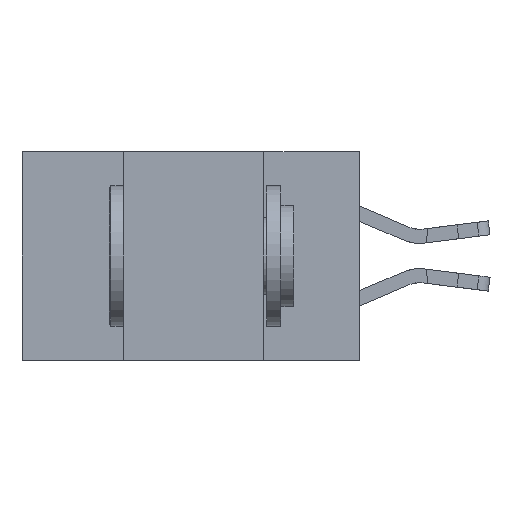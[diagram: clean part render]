
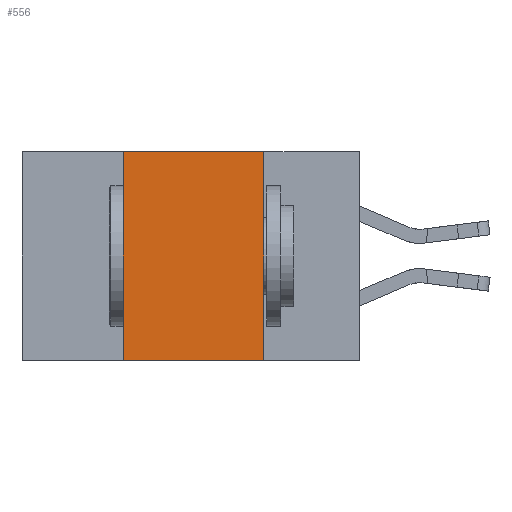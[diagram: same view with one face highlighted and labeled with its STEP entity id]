
A CAD part, left-side view. The second image highlights one B-rep face of the part: STEP entity #556.
In plain terms, the highlighted planar face has unit normal (-1, 0, 0).
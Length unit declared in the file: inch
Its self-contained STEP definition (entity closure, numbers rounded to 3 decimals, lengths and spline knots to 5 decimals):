
#209 = CARTESIAN_POINT ( 'NONE',  ( 0., 0.42, 0. ) ) ;
#556 = ADVANCED_FACE ( 'NONE', ( #5768 ), #14916, .F. ) ;
#893 = LINE ( 'NONE', #16815, #12955 ) ;
#2112 = LINE ( 'NONE', #15642, #14509 ) ;
#4511 = AXIS2_PLACEMENT_3D ( 'NONE', #15819, #16885, #16577 ) ;
#5581 = VECTOR ( 'NONE', #9529, 39.37008 ) ;
#5768 = FACE_OUTER_BOUND ( 'NONE', #12781, .T. ) ;
#6094 = VERTEX_POINT ( 'NONE', #17877 ) ;
#6844 = EDGE_CURVE ( 'NONE', #11597, #11289, #7750, .T. ) ;
#7247 = VECTOR ( 'NONE', #19493, 39.37008 ) ;
#7750 = LINE ( 'NONE', #18041, #7247 ) ;
#9408 = VERTEX_POINT ( 'NONE', #12818 ) ;
#9529 = DIRECTION ( 'NONE',  ( 0., -1., 0. ) ) ;
#10907 = ORIENTED_EDGE ( 'NONE', *, *, #16744, .F. ) ;
#11099 = ORIENTED_EDGE ( 'NONE', *, *, #6844, .F. ) ;
#11289 = VERTEX_POINT ( 'NONE', #16557 ) ;
#11597 = VERTEX_POINT ( 'NONE', #209 ) ;
#12057 = ORIENTED_EDGE ( 'NONE', *, *, #13238, .F. ) ;
#12228 = ORIENTED_EDGE ( 'NONE', *, *, #18544, .T. ) ;
#12781 = EDGE_LOOP ( 'NONE', ( #10907, #11099, #12057, #12228 ) ) ;
#12818 = CARTESIAN_POINT ( 'NONE',  ( 0., 0.17, -0.37 ) ) ;
#12955 = VECTOR ( 'NONE', #18255, 39.37008 ) ;
#13238 = EDGE_CURVE ( 'NONE', #6094, #11597, #893, .T. ) ;
#14509 = VECTOR ( 'NONE', #17101, 39.37008 ) ;
#14916 = PLANE ( 'NONE',  #4511 ) ;
#15331 = LINE ( 'NONE', #18339, #5581 ) ;
#15642 = CARTESIAN_POINT ( 'NONE',  ( 0., 0.17, 0. ) ) ;
#15819 = CARTESIAN_POINT ( 'NONE',  ( 0., 0.6, 0. ) ) ;
#16557 = CARTESIAN_POINT ( 'NONE',  ( 0., 0.17, 0. ) ) ;
#16577 = DIRECTION ( 'NONE',  ( 0., 0., -1. ) ) ;
#16744 = EDGE_CURVE ( 'NONE', #11289, #9408, #2112, .T. ) ;
#16815 = CARTESIAN_POINT ( 'NONE',  ( 0., 0.42, 0. ) ) ;
#16885 = DIRECTION ( 'NONE',  ( 1., 0., 0. ) ) ;
#17101 = DIRECTION ( 'NONE',  ( 0., 0., -1. ) ) ;
#17877 = CARTESIAN_POINT ( 'NONE',  ( 0., 0.42, -0.37 ) ) ;
#18041 = CARTESIAN_POINT ( 'NONE',  ( 0., 0.6, 0. ) ) ;
#18255 = DIRECTION ( 'NONE',  ( 0., 0., 1. ) ) ;
#18339 = CARTESIAN_POINT ( 'NONE',  ( 0., 0.6, -0.37 ) ) ;
#18544 = EDGE_CURVE ( 'NONE', #6094, #9408, #15331, .T. ) ;
#19493 = DIRECTION ( 'NONE',  ( 0., -1., 0. ) ) ;
